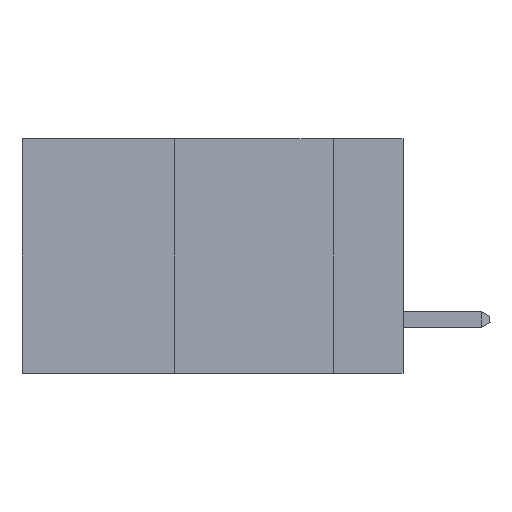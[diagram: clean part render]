
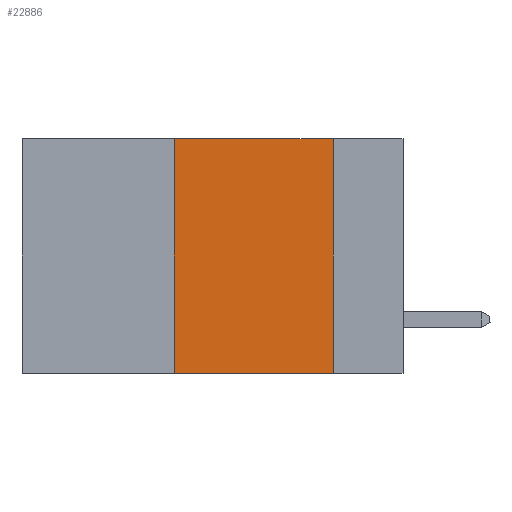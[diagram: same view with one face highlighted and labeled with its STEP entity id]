
A CAD part, left-side view. The second image highlights one B-rep face of the part: STEP entity #22886.
In plain terms, the highlighted planar face has unit normal (-1, 0, 0).
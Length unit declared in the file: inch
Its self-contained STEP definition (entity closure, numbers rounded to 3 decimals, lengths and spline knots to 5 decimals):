
#382 = ORIENTED_EDGE ( 'NONE', *, *, #1209, .F. ) ;
#1209 = EDGE_CURVE ( 'NONE', #22732, #14645, #23661, .T. ) ;
#2021 = DIRECTION ( 'NONE',  ( 0., -1., 0. ) ) ;
#2037 = VERTEX_POINT ( 'NONE', #20302 ) ;
#3204 = ORIENTED_EDGE ( 'NONE', *, *, #29807, .F. ) ;
#11093 = CARTESIAN_POINT ( 'NONE',  ( 0., 0.6, 0. ) ) ;
#12722 = EDGE_CURVE ( 'NONE', #2037, #26965, #31919, .T. ) ;
#13097 = DIRECTION ( 'NONE',  ( 0., 0., -1. ) ) ;
#13489 = DIRECTION ( 'NONE',  ( 1., 0., 0. ) ) ;
#14645 = VERTEX_POINT ( 'NONE', #36816 ) ;
#14792 = ORIENTED_EDGE ( 'NONE', *, *, #20097, .F. ) ;
#20097 = EDGE_CURVE ( 'NONE', #14645, #26965, #24850, .T. ) ;
#20111 = PLANE ( 'NONE',  #32879 ) ;
#20205 = CARTESIAN_POINT ( 'NONE',  ( 0., 0.36, 0. ) ) ;
#20302 = CARTESIAN_POINT ( 'NONE',  ( 0., 0.36, -0.37 ) ) ;
#20511 = CARTESIAN_POINT ( 'NONE',  ( 0., 0.11, -0.37 ) ) ;
#22276 = CARTESIAN_POINT ( 'NONE',  ( 0., 0.6, 0. ) ) ;
#22732 = VERTEX_POINT ( 'NONE', #26056 ) ;
#22886 = ADVANCED_FACE ( 'NONE', ( #26895 ), #20111, .F. ) ;
#22891 = VECTOR ( 'NONE', #26153, 39.37008 ) ;
#22995 = CARTESIAN_POINT ( 'NONE',  ( 0., 0.11, 0. ) ) ;
#23661 = LINE ( 'NONE', #11093, #33429 ) ;
#24850 = LINE ( 'NONE', #22995, #28115 ) ;
#25772 = CARTESIAN_POINT ( 'NONE',  ( 0., 0.6, -0.37 ) ) ;
#26056 = CARTESIAN_POINT ( 'NONE',  ( 0., 0.36, 0. ) ) ;
#26153 = DIRECTION ( 'NONE',  ( 0., 0., 1. ) ) ;
#26895 = FACE_OUTER_BOUND ( 'NONE', #37653, .T. ) ;
#26965 = VERTEX_POINT ( 'NONE', #20511 ) ;
#28115 = VECTOR ( 'NONE', #13097, 39.37008 ) ;
#29400 = LINE ( 'NONE', #20205, #22891 ) ;
#29593 = ORIENTED_EDGE ( 'NONE', *, *, #12722, .T. ) ;
#29807 = EDGE_CURVE ( 'NONE', #2037, #22732, #29400, .T. ) ;
#30956 = DIRECTION ( 'NONE',  ( 0., 0., -1. ) ) ;
#31513 = DIRECTION ( 'NONE',  ( 0., -1., 0. ) ) ;
#31919 = LINE ( 'NONE', #25772, #37544 ) ;
#32879 = AXIS2_PLACEMENT_3D ( 'NONE', #22276, #13489, #30956 ) ;
#33429 = VECTOR ( 'NONE', #31513, 39.37008 ) ;
#36816 = CARTESIAN_POINT ( 'NONE',  ( 0., 0.11, 0. ) ) ;
#37544 = VECTOR ( 'NONE', #2021, 39.37008 ) ;
#37653 = EDGE_LOOP ( 'NONE', ( #14792, #382, #3204, #29593 ) ) ;
